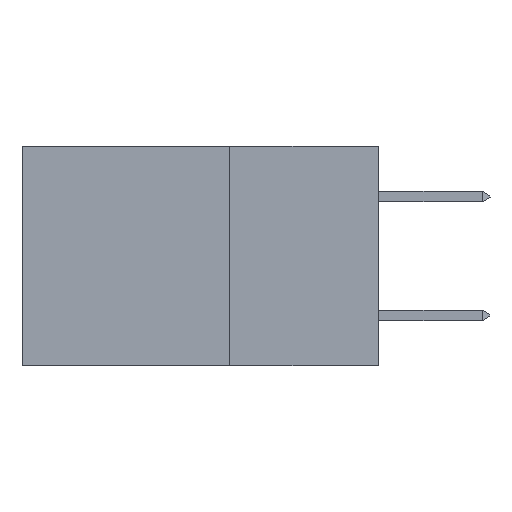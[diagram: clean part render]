
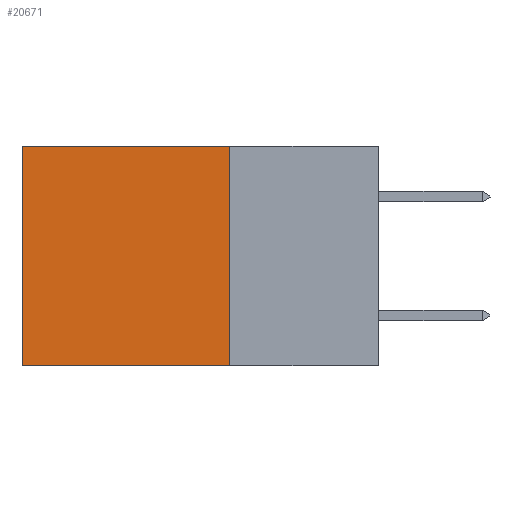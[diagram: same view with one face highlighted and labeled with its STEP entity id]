
A CAD part, left-side view. The second image highlights one B-rep face of the part: STEP entity #20671.
In plain terms, the highlighted planar face has unit normal (-1, 0, 0).
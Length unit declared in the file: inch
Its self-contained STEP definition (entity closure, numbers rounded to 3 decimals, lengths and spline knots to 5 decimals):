
#777 = EDGE_CURVE ( 'NONE', #4453, #19273, #14492, .T. ) ;
#2131 = LINE ( 'NONE', #16382, #22506 ) ;
#2565 = ORIENTED_EDGE ( 'NONE', *, *, #777, .T. ) ;
#3074 = CARTESIAN_POINT ( 'NONE',  ( 0.2615, 0.6, -0.37 ) ) ;
#3162 = DIRECTION ( 'NONE',  ( 0., 0., -1. ) ) ;
#3301 = VECTOR ( 'NONE', #26248, 39.37008 ) ;
#3526 = EDGE_CURVE ( 'NONE', #4453, #11426, #19639, .T. ) ;
#4157 = FACE_OUTER_BOUND ( 'NONE', #13087, .T. ) ;
#4453 = VERTEX_POINT ( 'NONE', #19035 ) ;
#5464 = VERTEX_POINT ( 'NONE', #3074 ) ;
#5718 = DIRECTION ( 'NONE',  ( 1., 0., 0. ) ) ;
#7681 = ORIENTED_EDGE ( 'NONE', *, *, #16735, .T. ) ;
#7685 = CARTESIAN_POINT ( 'NONE',  ( 0.2615, 0.25, -0.37 ) ) ;
#7730 = LINE ( 'NONE', #10162, #13355 ) ;
#7787 = AXIS2_PLACEMENT_3D ( 'NONE', #18324, #5718, #20422 ) ;
#10162 = CARTESIAN_POINT ( 'NONE',  ( 0.2615, 0.6, -0.37 ) ) ;
#10420 = VECTOR ( 'NONE', #3162, 39.37008 ) ;
#10952 = EDGE_CURVE ( 'NONE', #11426, #5464, #2131, .T. ) ;
#11426 = VERTEX_POINT ( 'NONE', #7685 ) ;
#11963 = PLANE ( 'NONE',  #7787 ) ;
#13087 = EDGE_LOOP ( 'NONE', ( #7681, #16658, #27020, #2565 ) ) ;
#13355 = VECTOR ( 'NONE', #22751, 39.37008 ) ;
#13658 = CARTESIAN_POINT ( 'NONE',  ( 0.2615, 0.25, -0.37 ) ) ;
#14492 = LINE ( 'NONE', #26936, #3301 ) ;
#16382 = CARTESIAN_POINT ( 'NONE',  ( 0.2615, 0.25, -0.37 ) ) ;
#16658 = ORIENTED_EDGE ( 'NONE', *, *, #10952, .F. ) ;
#16735 = EDGE_CURVE ( 'NONE', #19273, #5464, #7730, .T. ) ;
#18324 = CARTESIAN_POINT ( 'NONE',  ( 0.2615, 0.25, -0.37 ) ) ;
#19035 = CARTESIAN_POINT ( 'NONE',  ( 0.2615, 0.25, 0. ) ) ;
#19273 = VERTEX_POINT ( 'NONE', #22594 ) ;
#19639 = LINE ( 'NONE', #13658, #10420 ) ;
#20422 = DIRECTION ( 'NONE',  ( 0., 0., -1. ) ) ;
#20671 = ADVANCED_FACE ( 'NONE', ( #4157 ), #11963, .F. ) ;
#22506 = VECTOR ( 'NONE', #26791, 39.37008 ) ;
#22594 = CARTESIAN_POINT ( 'NONE',  ( 0.2615, 0.6, 0. ) ) ;
#22751 = DIRECTION ( 'NONE',  ( 0., 0., -1. ) ) ;
#26248 = DIRECTION ( 'NONE',  ( 0., 1., 0. ) ) ;
#26791 = DIRECTION ( 'NONE',  ( 0., 1., 0. ) ) ;
#26936 = CARTESIAN_POINT ( 'NONE',  ( 0.2615, 0.25, 0. ) ) ;
#27020 = ORIENTED_EDGE ( 'NONE', *, *, #3526, .F. ) ;
